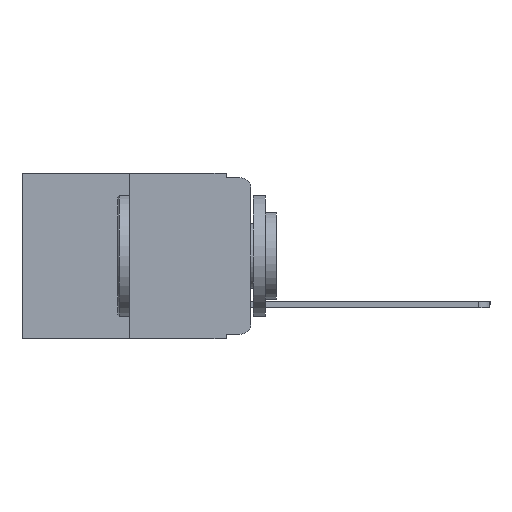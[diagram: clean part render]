
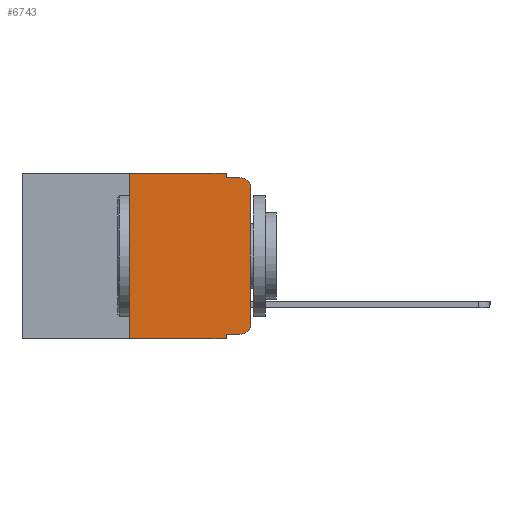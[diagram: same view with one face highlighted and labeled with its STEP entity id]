
A CAD part, left-side view. The second image highlights one B-rep face of the part: STEP entity #6743.
In plain terms, the highlighted planar face has unit normal (-1, 0, 0).
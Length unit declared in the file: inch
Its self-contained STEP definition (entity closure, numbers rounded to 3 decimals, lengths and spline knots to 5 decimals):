
#191 = DIRECTION ( 'NONE',  ( 0., 0., -1. ) ) ;
#456 = DIRECTION ( 'NONE',  ( 0., -1., 0. ) ) ;
#579 = DIRECTION ( 'NONE',  ( 0., 0., -1. ) ) ;
#852 = VECTOR ( 'NONE', #191, 39.37008 ) ;
#932 = CARTESIAN_POINT ( 'NONE',  ( 0., 0., 0. ) ) ;
#1385 = VERTEX_POINT ( 'NONE', #12955 ) ;
#1660 = VERTEX_POINT ( 'NONE', #10197 ) ;
#2215 = VERTEX_POINT ( 'NONE', #4565 ) ;
#2479 = CARTESIAN_POINT ( 'NONE',  ( 0., 0.051, 0. ) ) ;
#2626 = DIRECTION ( 'NONE',  ( 0., -1., 0. ) ) ;
#2932 = CARTESIAN_POINT ( 'NONE',  ( 0., 0.051, -0.01 ) ) ;
#2994 = EDGE_CURVE ( 'NONE', #4917, #19158, #15652, .T. ) ;
#3055 = ORIENTED_EDGE ( 'NONE', *, *, #18176, .T. ) ;
#3166 = LINE ( 'NONE', #15175, #852 ) ;
#3540 = LINE ( 'NONE', #5489, #16115 ) ;
#3649 = VECTOR ( 'NONE', #17857, 39.37008 ) ;
#3677 = CARTESIAN_POINT ( 'NONE',  ( 0., 0.051, -0.333 ) ) ;
#3970 = EDGE_CURVE ( 'NONE', #19158, #11646, #3540, .T. ) ;
#4078 = DIRECTION ( 'NONE',  ( 1., 0., 0. ) ) ;
#4279 = DIRECTION ( 'NONE',  ( 0., 0., 1. ) ) ;
#4341 = LINE ( 'NONE', #2932, #15866 ) ;
#4565 = CARTESIAN_POINT ( 'NONE',  ( 0., 0.051, -0.01 ) ) ;
#4682 = LINE ( 'NONE', #9190, #18340 ) ;
#4683 = VECTOR ( 'NONE', #19968, 39.37008 ) ;
#4917 = VERTEX_POINT ( 'NONE', #12985 ) ;
#4947 = CARTESIAN_POINT ( 'NONE',  ( 0., 0., -0.313 ) ) ;
#4991 = CARTESIAN_POINT ( 'NONE',  ( 0., 0.25, 0. ) ) ;
#5489 = CARTESIAN_POINT ( 'NONE',  ( 0., 0.473, 0. ) ) ;
#6480 = CARTESIAN_POINT ( 'NONE',  ( 0., 0.051, -0.343 ) ) ;
#6557 = DIRECTION ( 'NONE',  ( 0., 0., -1. ) ) ;
#6743 = ADVANCED_FACE ( 'NONE', ( #19171 ), #18836, .F. ) ;
#7009 = CARTESIAN_POINT ( 'NONE',  ( 0., 0.02, -0.313 ) ) ;
#7465 = VERTEX_POINT ( 'NONE', #3677 ) ;
#8277 = EDGE_CURVE ( 'NONE', #4917, #20934, #11196, .T. ) ;
#8697 = ORIENTED_EDGE ( 'NONE', *, *, #17486, .F. ) ;
#8835 = VERTEX_POINT ( 'NONE', #4947 ) ;
#9190 = CARTESIAN_POINT ( 'NONE',  ( 0., 0.051, -0.333 ) ) ;
#9548 = DIRECTION ( 'NONE',  ( -1., 0., 0. ) ) ;
#9586 = EDGE_CURVE ( 'NONE', #7465, #11080, #4682, .T. ) ;
#9611 = DIRECTION ( 'NONE',  ( 0., -1., 0. ) ) ;
#9614 = AXIS2_PLACEMENT_3D ( 'NONE', #7009, #13458, #20132 ) ;
#10197 = CARTESIAN_POINT ( 'NONE',  ( 0., 0.02, -0.01 ) ) ;
#10235 = CARTESIAN_POINT ( 'NONE',  ( 0., 0.051, 0. ) ) ;
#10427 = ORIENTED_EDGE ( 'NONE', *, *, #18341, .T. ) ;
#10623 = CARTESIAN_POINT ( 'NONE',  ( 0., 0.25, 0. ) ) ;
#11080 = VERTEX_POINT ( 'NONE', #15287 ) ;
#11196 = LINE ( 'NONE', #19606, #3649 ) ;
#11518 = LINE ( 'NONE', #932, #14474 ) ;
#11646 = VERTEX_POINT ( 'NONE', #2479 ) ;
#11888 = LINE ( 'NONE', #10235, #4683 ) ;
#12355 = ORIENTED_EDGE ( 'NONE', *, *, #17875, .F. ) ;
#12507 = ORIENTED_EDGE ( 'NONE', *, *, #3970, .F. ) ;
#12680 = AXIS2_PLACEMENT_3D ( 'NONE', #13809, #4078, #579 ) ;
#12955 = CARTESIAN_POINT ( 'NONE',  ( 0., 0., -0.03 ) ) ;
#12985 = CARTESIAN_POINT ( 'NONE',  ( 0., 0.25, -0.343 ) ) ;
#13236 = CARTESIAN_POINT ( 'NONE',  ( 0., 0.02, -0.03 ) ) ;
#13458 = DIRECTION ( 'NONE',  ( -1., 0., 0. ) ) ;
#13555 = EDGE_CURVE ( 'NONE', #1385, #1660, #18441, .T. ) ;
#13809 = CARTESIAN_POINT ( 'NONE',  ( 0., 0.473, 0. ) ) ;
#14474 = VECTOR ( 'NONE', #16135, 39.37008 ) ;
#14619 = ORIENTED_EDGE ( 'NONE', *, *, #2994, .F. ) ;
#15175 = CARTESIAN_POINT ( 'NONE',  ( 0., 0.051, 0. ) ) ;
#15287 = CARTESIAN_POINT ( 'NONE',  ( 0., 0.02, -0.333 ) ) ;
#15652 = LINE ( 'NONE', #10623, #16389 ) ;
#15866 = VECTOR ( 'NONE', #9611, 39.37008 ) ;
#15884 = CIRCLE ( 'NONE', #9614, 0.02 ) ;
#16115 = VECTOR ( 'NONE', #456, 39.37008 ) ;
#16121 = EDGE_LOOP ( 'NONE', ( #3055, #17177, #19837, #12355, #12507, #14619, #17306, #8697, #16446, #10427 ) ) ;
#16135 = DIRECTION ( 'NONE',  ( 0., 0., 1. ) ) ;
#16389 = VECTOR ( 'NONE', #4279, 39.37008 ) ;
#16446 = ORIENTED_EDGE ( 'NONE', *, *, #9586, .T. ) ;
#17177 = ORIENTED_EDGE ( 'NONE', *, *, #13555, .T. ) ;
#17306 = ORIENTED_EDGE ( 'NONE', *, *, #8277, .T. ) ;
#17486 = EDGE_CURVE ( 'NONE', #7465, #20934, #3166, .T. ) ;
#17785 = EDGE_CURVE ( 'NONE', #2215, #1660, #4341, .T. ) ;
#17857 = DIRECTION ( 'NONE',  ( 0., -1., 0. ) ) ;
#17875 = EDGE_CURVE ( 'NONE', #11646, #2215, #11888, .T. ) ;
#18176 = EDGE_CURVE ( 'NONE', #8835, #1385, #11518, .T. ) ;
#18340 = VECTOR ( 'NONE', #2626, 39.37008 ) ;
#18341 = EDGE_CURVE ( 'NONE', #11080, #8835, #15884, .T. ) ;
#18441 = CIRCLE ( 'NONE', #18792, 0.02 ) ;
#18792 = AXIS2_PLACEMENT_3D ( 'NONE', #13236, #9548, #6557 ) ;
#18836 = PLANE ( 'NONE',  #12680 ) ;
#19158 = VERTEX_POINT ( 'NONE', #4991 ) ;
#19171 = FACE_OUTER_BOUND ( 'NONE', #16121, .T. ) ;
#19606 = CARTESIAN_POINT ( 'NONE',  ( 0., 0.473, -0.343 ) ) ;
#19837 = ORIENTED_EDGE ( 'NONE', *, *, #17785, .F. ) ;
#19968 = DIRECTION ( 'NONE',  ( 0., 0., -1. ) ) ;
#20132 = DIRECTION ( 'NONE',  ( 0., 0., -1. ) ) ;
#20934 = VERTEX_POINT ( 'NONE', #6480 ) ;
